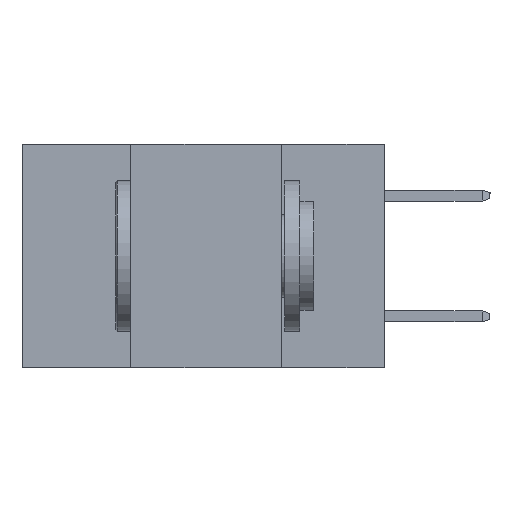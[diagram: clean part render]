
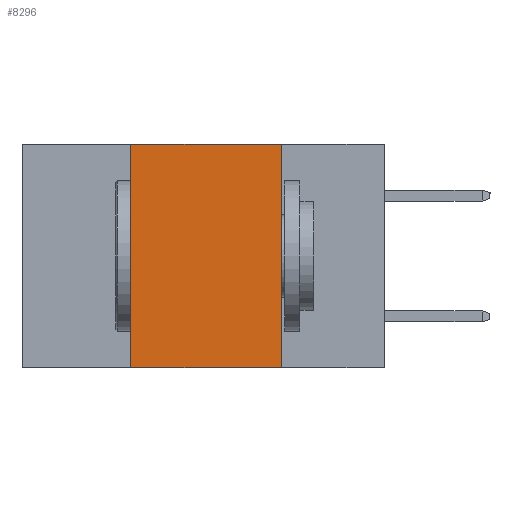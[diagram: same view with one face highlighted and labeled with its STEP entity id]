
A CAD part, left-side view. The second image highlights one B-rep face of the part: STEP entity #8296.
In plain terms, the highlighted planar face has unit normal (-1, 0, 0).
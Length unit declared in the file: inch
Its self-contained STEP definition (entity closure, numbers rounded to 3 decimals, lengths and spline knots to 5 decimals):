
#569 = CARTESIAN_POINT ( 'NONE',  ( 0., 0.17, -0.37 ) ) ;
#700 = DIRECTION ( 'NONE',  ( 0., 0., -1. ) ) ;
#1349 = VERTEX_POINT ( 'NONE', #8192 ) ;
#1667 = DIRECTION ( 'NONE',  ( 0., -1., 0. ) ) ;
#1745 = DIRECTION ( 'NONE',  ( 0., 0., -1. ) ) ;
#3145 = VERTEX_POINT ( 'NONE', #3936 ) ;
#3603 = EDGE_CURVE ( 'NONE', #1349, #5146, #8021, .T. ) ;
#3788 = PLANE ( 'NONE',  #3914 ) ;
#3914 = AXIS2_PLACEMENT_3D ( 'NONE', #7955, #10066, #700 ) ;
#3936 = CARTESIAN_POINT ( 'NONE',  ( 0., 0.42, 0. ) ) ;
#3979 = CARTESIAN_POINT ( 'NONE',  ( 0., 0.6, 0. ) ) ;
#4562 = EDGE_CURVE ( 'NONE', #8731, #3145, #10990, .T. ) ;
#4708 = DIRECTION ( 'NONE',  ( 0., 0., 1. ) ) ;
#4874 = ORIENTED_EDGE ( 'NONE', *, *, #3603, .F. ) ;
#5095 = LINE ( 'NONE', #11490, #8136 ) ;
#5146 = VERTEX_POINT ( 'NONE', #5848 ) ;
#5600 = CARTESIAN_POINT ( 'NONE',  ( 0., 0.42, -0.37 ) ) ;
#5636 = EDGE_CURVE ( 'NONE', #3145, #1349, #9045, .T. ) ;
#5848 = CARTESIAN_POINT ( 'NONE',  ( 0., 0.17, -0.37 ) ) ;
#6043 = ORIENTED_EDGE ( 'NONE', *, *, #5636, .F. ) ;
#6093 = VECTOR ( 'NONE', #1667, 39.37008 ) ;
#7134 = DIRECTION ( 'NONE',  ( 0., -1., 0. ) ) ;
#7221 = ORIENTED_EDGE ( 'NONE', *, *, #12227, .T. ) ;
#7823 = VECTOR ( 'NONE', #4708, 39.37008 ) ;
#7955 = CARTESIAN_POINT ( 'NONE',  ( 0., 0.6, 0. ) ) ;
#8021 = LINE ( 'NONE', #569, #8665 ) ;
#8136 = VECTOR ( 'NONE', #7134, 39.37008 ) ;
#8192 = CARTESIAN_POINT ( 'NONE',  ( 0., 0.17, 0. ) ) ;
#8296 = ADVANCED_FACE ( 'NONE', ( #13332 ), #3788, .F. ) ;
#8665 = VECTOR ( 'NONE', #1745, 39.37008 ) ;
#8731 = VERTEX_POINT ( 'NONE', #12715 ) ;
#8748 = EDGE_LOOP ( 'NONE', ( #4874, #6043, #8853, #7221 ) ) ;
#8853 = ORIENTED_EDGE ( 'NONE', *, *, #4562, .F. ) ;
#9045 = LINE ( 'NONE', #3979, #6093 ) ;
#10066 = DIRECTION ( 'NONE',  ( 1., 0., 0. ) ) ;
#10990 = LINE ( 'NONE', #5600, #7823 ) ;
#11490 = CARTESIAN_POINT ( 'NONE',  ( 0., 0.6, -0.37 ) ) ;
#12227 = EDGE_CURVE ( 'NONE', #8731, #5146, #5095, .T. ) ;
#12715 = CARTESIAN_POINT ( 'NONE',  ( 0., 0.42, -0.37 ) ) ;
#13332 = FACE_OUTER_BOUND ( 'NONE', #8748, .T. ) ;
